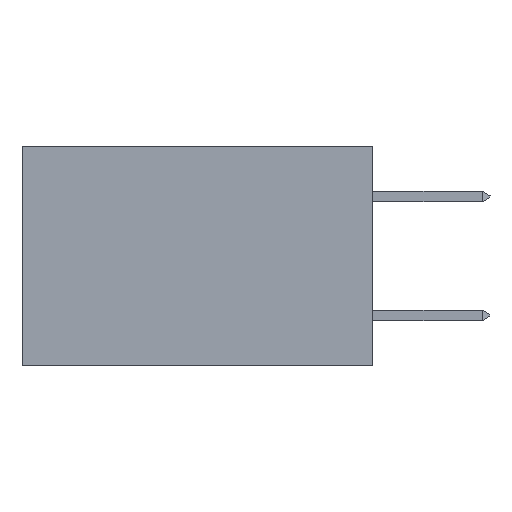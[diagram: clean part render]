
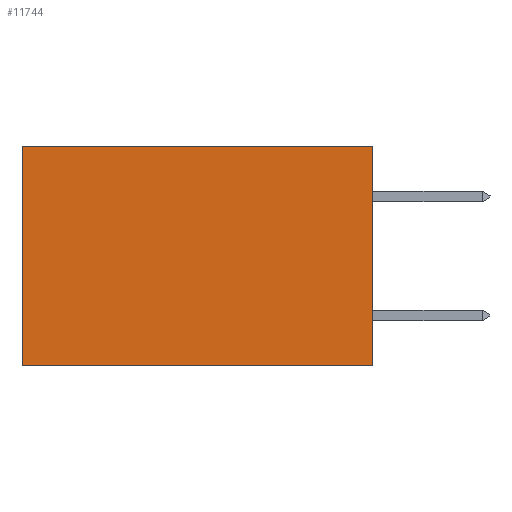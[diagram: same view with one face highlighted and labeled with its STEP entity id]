
A CAD part, left-side view. The second image highlights one B-rep face of the part: STEP entity #11744.
In plain terms, the highlighted planar face has unit normal (-1, 0, 0).
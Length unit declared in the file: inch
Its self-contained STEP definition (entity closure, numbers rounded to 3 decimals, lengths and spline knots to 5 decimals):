
#572 = VERTEX_POINT ( 'NONE', #14958 ) ;
#1054 = CARTESIAN_POINT ( 'NONE',  ( 0.277, 0.59, 0. ) ) ;
#1396 = DIRECTION ( 'NONE',  ( 0., 0., -1. ) ) ;
#1523 = EDGE_CURVE ( 'NONE', #8378, #572, #7267, .T. ) ;
#1768 = CARTESIAN_POINT ( 'NONE',  ( 0.277, 0., -0.37 ) ) ;
#1808 = LINE ( 'NONE', #10914, #15366 ) ;
#2615 = ORIENTED_EDGE ( 'NONE', *, *, #17730, .F. ) ;
#4430 = DIRECTION ( 'NONE',  ( 0., 1., 0. ) ) ;
#4981 = ORIENTED_EDGE ( 'NONE', *, *, #16312, .T. ) ;
#5213 = VERTEX_POINT ( 'NONE', #23246 ) ;
#6839 = VECTOR ( 'NONE', #21904, 39.37008 ) ;
#7267 = LINE ( 'NONE', #1768, #12139 ) ;
#7276 = VERTEX_POINT ( 'NONE', #1054 ) ;
#8378 = VERTEX_POINT ( 'NONE', #14434 ) ;
#8633 = EDGE_CURVE ( 'NONE', #8378, #7276, #18610, .T. ) ;
#9323 = EDGE_LOOP ( 'NONE', ( #4981, #2615, #13748, #15249 ) ) ;
#10914 = CARTESIAN_POINT ( 'NONE',  ( 0.277, 0., -0.37 ) ) ;
#11002 = CARTESIAN_POINT ( 'NONE',  ( 0.277, 0., -0.37 ) ) ;
#11720 = LINE ( 'NONE', #18285, #6839 ) ;
#11744 = ADVANCED_FACE ( 'NONE', ( #13531 ), #23593, .F. ) ;
#11839 = AXIS2_PLACEMENT_3D ( 'NONE', #11002, #23661, #12832 ) ;
#12139 = VECTOR ( 'NONE', #1396, 39.37008 ) ;
#12832 = DIRECTION ( 'NONE',  ( 0., 0., -1. ) ) ;
#13531 = FACE_OUTER_BOUND ( 'NONE', #9323, .T. ) ;
#13562 = CARTESIAN_POINT ( 'NONE',  ( 0.277, 0., 0. ) ) ;
#13748 = ORIENTED_EDGE ( 'NONE', *, *, #1523, .F. ) ;
#14247 = VECTOR ( 'NONE', #4430, 39.37008 ) ;
#14434 = CARTESIAN_POINT ( 'NONE',  ( 0.277, 0., 0. ) ) ;
#14958 = CARTESIAN_POINT ( 'NONE',  ( 0.277, 0., -0.37 ) ) ;
#15249 = ORIENTED_EDGE ( 'NONE', *, *, #8633, .T. ) ;
#15366 = VECTOR ( 'NONE', #16350, 39.37008 ) ;
#16312 = EDGE_CURVE ( 'NONE', #7276, #5213, #11720, .T. ) ;
#16350 = DIRECTION ( 'NONE',  ( 0., 1., 0. ) ) ;
#17730 = EDGE_CURVE ( 'NONE', #572, #5213, #1808, .T. ) ;
#18285 = CARTESIAN_POINT ( 'NONE',  ( 0.277, 0.59, -0.37 ) ) ;
#18610 = LINE ( 'NONE', #13562, #14247 ) ;
#21904 = DIRECTION ( 'NONE',  ( 0., 0., -1. ) ) ;
#23246 = CARTESIAN_POINT ( 'NONE',  ( 0.277, 0.59, -0.37 ) ) ;
#23593 = PLANE ( 'NONE',  #11839 ) ;
#23661 = DIRECTION ( 'NONE',  ( 1., 0., 0. ) ) ;
